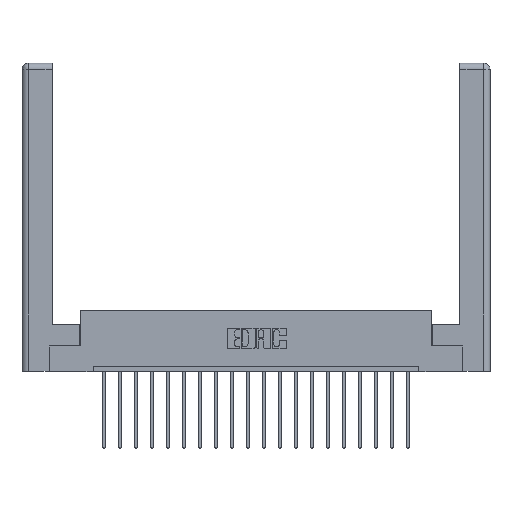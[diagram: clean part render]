
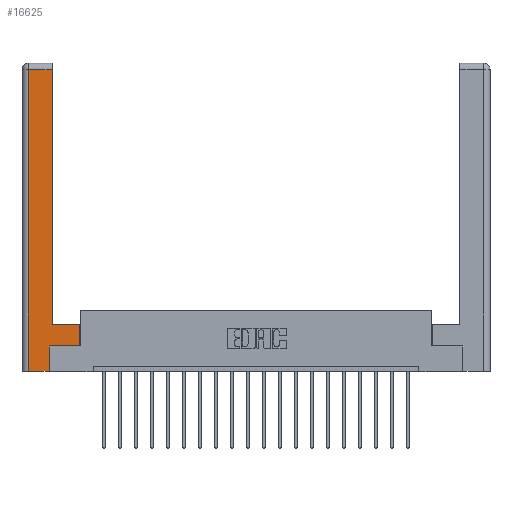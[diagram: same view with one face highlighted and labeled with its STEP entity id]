
A CAD part, top view. The second image highlights one B-rep face of the part: STEP entity #16625.
In plain terms, the highlighted planar face has unit normal (0, 0, 1).
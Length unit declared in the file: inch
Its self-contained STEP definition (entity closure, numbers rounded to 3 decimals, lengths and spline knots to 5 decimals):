
#197 = LINE ( 'NONE', #12328, #3852 ) ;
#958 = CARTESIAN_POINT ( 'NONE',  ( 0.265, 0., 0. ) ) ;
#988 = EDGE_CURVE ( 'NONE', #4677, #5754, #5894, .T. ) ;
#1547 = ORIENTED_EDGE ( 'NONE', *, *, #988, .T. ) ;
#1706 = VECTOR ( 'NONE', #14191, 39.37008 ) ;
#2032 = VERTEX_POINT ( 'NONE', #10990 ) ;
#2243 = DIRECTION ( 'NONE',  ( 0., 1., 0. ) ) ;
#2772 = ORIENTED_EDGE ( 'NONE', *, *, #8981, .T. ) ;
#2898 = DIRECTION ( 'NONE',  ( -1., 0., 0. ) ) ;
#2980 = CARTESIAN_POINT ( 'NONE',  ( 0.0615, 0., 0. ) ) ;
#3236 = CARTESIAN_POINT ( 'NONE',  ( 0.565, 0.45, 0. ) ) ;
#3264 = CARTESIAN_POINT ( 'NONE',  ( 0.265, 0.245, 0. ) ) ;
#3329 = DIRECTION ( 'NONE',  ( 0., 1., 0. ) ) ;
#3574 = VECTOR ( 'NONE', #13815, 39.37008 ) ;
#3852 = VECTOR ( 'NONE', #2898, 39.37008 ) ;
#4377 = AXIS2_PLACEMENT_3D ( 'NONE', #10743, #7670, #13802 ) ;
#4420 = VERTEX_POINT ( 'NONE', #12817 ) ;
#4601 = ORIENTED_EDGE ( 'NONE', *, *, #16789, .T. ) ;
#4677 = VERTEX_POINT ( 'NONE', #13827 ) ;
#5189 = CARTESIAN_POINT ( 'NONE',  ( 0.295, 2.94, 0. ) ) ;
#5231 = CARTESIAN_POINT ( 'NONE',  ( 0.295, 3., 0. ) ) ;
#5754 = VERTEX_POINT ( 'NONE', #3236 ) ;
#5894 = LINE ( 'NONE', #12596, #1706 ) ;
#5972 = EDGE_LOOP ( 'NONE', ( #18080, #4601, #2772, #6737, #8568, #10448, #1547, #16413 ) ) ;
#6737 = ORIENTED_EDGE ( 'NONE', *, *, #9088, .T. ) ;
#6935 = EDGE_CURVE ( 'NONE', #15737, #4677, #16465, .T. ) ;
#7163 = EDGE_CURVE ( 'NONE', #4420, #8514, #16930, .T. ) ;
#7670 = DIRECTION ( 'NONE',  ( 0., 0., -1. ) ) ;
#8087 = EDGE_CURVE ( 'NONE', #5754, #4420, #19655, .T. ) ;
#8514 = VERTEX_POINT ( 'NONE', #5189 ) ;
#8516 = VERTEX_POINT ( 'NONE', #14675 ) ;
#8568 = ORIENTED_EDGE ( 'NONE', *, *, #12419, .T. ) ;
#8838 = CARTESIAN_POINT ( 'NONE',  ( 0.265, 0.245, 0. ) ) ;
#8981 = EDGE_CURVE ( 'NONE', #8516, #2032, #17114, .T. ) ;
#9088 = EDGE_CURVE ( 'NONE', #2032, #11099, #18855, .T. ) ;
#9126 = VECTOR ( 'NONE', #3329, 39.37008 ) ;
#10448 = ORIENTED_EDGE ( 'NONE', *, *, #6935, .T. ) ;
#10601 = PLANE ( 'NONE',  #4377 ) ;
#10743 = CARTESIAN_POINT ( 'NONE',  ( 0., 0., 0. ) ) ;
#10878 = DIRECTION ( 'NONE',  ( 1., 0., 0. ) ) ;
#10990 = CARTESIAN_POINT ( 'NONE',  ( 0.0615, 0., 0. ) ) ;
#11099 = VERTEX_POINT ( 'NONE', #958 ) ;
#11906 = VECTOR ( 'NONE', #10878, 39.37008 ) ;
#12328 = CARTESIAN_POINT ( 'NONE',  ( 0.0615, 2.94, 0. ) ) ;
#12419 = EDGE_CURVE ( 'NONE', #11099, #15737, #17475, .T. ) ;
#12596 = CARTESIAN_POINT ( 'NONE',  ( 0.565, 0.45, 0. ) ) ;
#12645 = CARTESIAN_POINT ( 'NONE',  ( 0.565, 0.245, 0. ) ) ;
#12739 = VECTOR ( 'NONE', #2243, 39.37008 ) ;
#12817 = CARTESIAN_POINT ( 'NONE',  ( 0.295, 0.45, 0. ) ) ;
#12917 = VECTOR ( 'NONE', #13793, 39.37008 ) ;
#12954 = FACE_OUTER_BOUND ( 'NONE', #5972, .T. ) ;
#12966 = DIRECTION ( 'NONE',  ( 1., 0., 0. ) ) ;
#13793 = DIRECTION ( 'NONE',  ( 0., -1., 0. ) ) ;
#13802 = DIRECTION ( 'NONE',  ( -1., 0., 0. ) ) ;
#13815 = DIRECTION ( 'NONE',  ( -1., 0., 0. ) ) ;
#13827 = CARTESIAN_POINT ( 'NONE',  ( 0.565, 0.245, 0. ) ) ;
#14191 = DIRECTION ( 'NONE',  ( 0., 1., 0. ) ) ;
#14675 = CARTESIAN_POINT ( 'NONE',  ( 0.0615, 2.94, 0. ) ) ;
#15737 = VERTEX_POINT ( 'NONE', #8838 ) ;
#16413 = ORIENTED_EDGE ( 'NONE', *, *, #8087, .T. ) ;
#16465 = LINE ( 'NONE', #12645, #16706 ) ;
#16625 = ADVANCED_FACE ( 'NONE', ( #12954 ), #10601, .F. ) ;
#16706 = VECTOR ( 'NONE', #12966, 39.37008 ) ;
#16789 = EDGE_CURVE ( 'NONE', #8514, #8516, #197, .T. ) ;
#16930 = LINE ( 'NONE', #5231, #12739 ) ;
#17114 = LINE ( 'NONE', #2980, #12917 ) ;
#17475 = LINE ( 'NONE', #3264, #9126 ) ;
#18080 = ORIENTED_EDGE ( 'NONE', *, *, #7163, .T. ) ;
#18599 = CARTESIAN_POINT ( 'NONE',  ( 0.295, 0.45, 0. ) ) ;
#18716 = CARTESIAN_POINT ( 'NONE',  ( 0.265, 0., 0. ) ) ;
#18855 = LINE ( 'NONE', #18716, #11906 ) ;
#19655 = LINE ( 'NONE', #18599, #3574 ) ;
